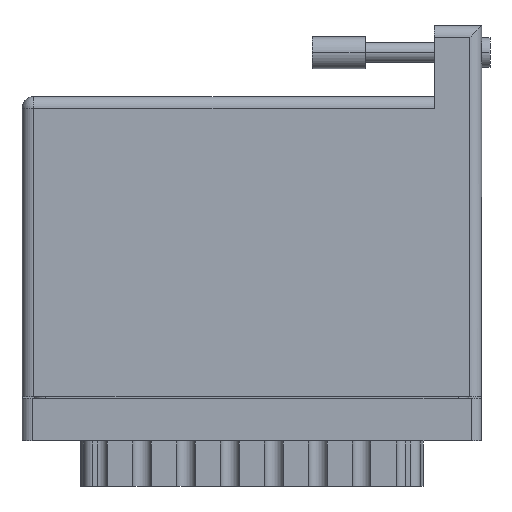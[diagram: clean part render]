
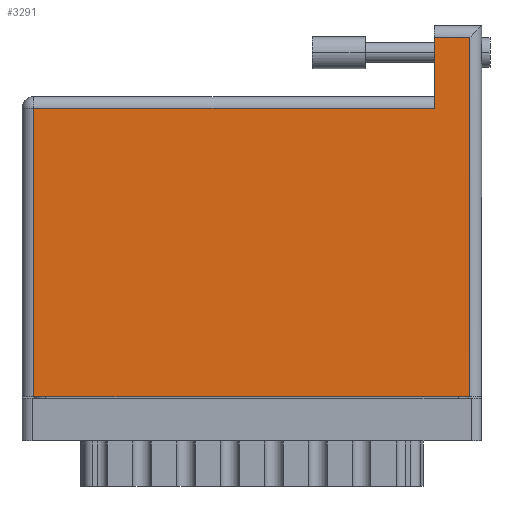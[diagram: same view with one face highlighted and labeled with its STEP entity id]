
A CAD part, front view. The second image highlights one B-rep face of the part: STEP entity #3291.
In plain terms, the highlighted face is planar.
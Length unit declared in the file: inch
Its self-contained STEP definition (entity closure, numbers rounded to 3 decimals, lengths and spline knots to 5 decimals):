
#130 = DIRECTION ( 'NONE',  ( -1., 0., 0. ) ) ;
#2239 = ORIENTED_EDGE ( 'NONE', *, *, #59741, .T. ) ;
#3291 = ADVANCED_FACE ( 'NONE', ( #67220 ), #52485, .F. ) ;
#6476 = CARTESIAN_POINT ( 'NONE',  ( 2.648, 0., 0. ) ) ;
#7361 = DIRECTION ( 'NONE',  ( 0., 0., -1. ) ) ;
#7433 = EDGE_LOOP ( 'NONE', ( #57592, #58185, #2239, #50515, #8734, #17443 ) ) ;
#8734 = ORIENTED_EDGE ( 'NONE', *, *, #58323, .T. ) ;
#8827 = EDGE_CURVE ( 'NONE', #49490, #54449, #51540, .T. ) ;
#10073 = CARTESIAN_POINT ( 'NONE',  ( 0., 1.705, 0. ) ) ;
#11583 = VERTEX_POINT ( 'NONE', #41017 ) ;
#15685 = DIRECTION ( 'NONE',  ( 0., -1., 0. ) ) ;
#17443 = ORIENTED_EDGE ( 'NONE', *, *, #55694, .T. ) ;
#17462 = EDGE_CURVE ( 'NONE', #61643, #49490, #47415, .T. ) ;
#17784 = DIRECTION ( 'NONE',  ( -1., 0., 0. ) ) ;
#19497 = EDGE_CURVE ( 'NONE', #45584, #11583, #55218, .T. ) ;
#20700 = VERTEX_POINT ( 'NONE', #58677 ) ;
#23329 = CARTESIAN_POINT ( 'NONE',  ( 0., 0., 0. ) ) ;
#23702 = LINE ( 'NONE', #65901, #54488 ) ;
#24988 = CARTESIAN_POINT ( 'NONE',  ( 0.07, 0., 0. ) ) ;
#28035 = VECTOR ( 'NONE', #15685, 39.37008 ) ;
#28466 = VECTOR ( 'NONE', #66991, 39.37008 ) ;
#31326 = CARTESIAN_POINT ( 'NONE',  ( 0.07, 0., 0. ) ) ;
#39415 = VECTOR ( 'NONE', #63774, 39.37008 ) ;
#41017 = CARTESIAN_POINT ( 'NONE',  ( 2.648, 2.125, 0. ) ) ;
#41182 = CARTESIAN_POINT ( 'NONE',  ( 2.438, 1.705, 0. ) ) ;
#42719 = CARTESIAN_POINT ( 'NONE',  ( 2.438, 2.195, 0. ) ) ;
#43372 = CARTESIAN_POINT ( 'NONE',  ( 0., 1.775, 0. ) ) ;
#44126 = DIRECTION ( 'NONE',  ( 1., 0., 0. ) ) ;
#45584 = VERTEX_POINT ( 'NONE', #6476 ) ;
#47415 = LINE ( 'NONE', #10073, #65191 ) ;
#48320 = LINE ( 'NONE', #42719, #39415 ) ;
#49490 = VERTEX_POINT ( 'NONE', #54366 ) ;
#50515 = ORIENTED_EDGE ( 'NONE', *, *, #19497, .T. ) ;
#51127 = LINE ( 'NONE', #23329, #64134 ) ;
#51540 = LINE ( 'NONE', #31326, #28035 ) ;
#52485 = PLANE ( 'NONE',  #66980 ) ;
#54366 = CARTESIAN_POINT ( 'NONE',  ( 0.07, 1.705, 0. ) ) ;
#54449 = VERTEX_POINT ( 'NONE', #24988 ) ;
#54488 = VECTOR ( 'NONE', #60951, 39.37008 ) ;
#55218 = LINE ( 'NONE', #61777, #28466 ) ;
#55694 = EDGE_CURVE ( 'NONE', #20700, #61643, #48320, .T. ) ;
#57592 = ORIENTED_EDGE ( 'NONE', *, *, #17462, .T. ) ;
#58185 = ORIENTED_EDGE ( 'NONE', *, *, #8827, .T. ) ;
#58323 = EDGE_CURVE ( 'NONE', #11583, #20700, #23702, .T. ) ;
#58677 = CARTESIAN_POINT ( 'NONE',  ( 2.438, 2.125, 0. ) ) ;
#59741 = EDGE_CURVE ( 'NONE', #54449, #45584, #51127, .T. ) ;
#60951 = DIRECTION ( 'NONE',  ( -1., 0., 0. ) ) ;
#61643 = VERTEX_POINT ( 'NONE', #41182 ) ;
#61777 = CARTESIAN_POINT ( 'NONE',  ( 2.648, 2.195, 0. ) ) ;
#63774 = DIRECTION ( 'NONE',  ( 0., -1., 0. ) ) ;
#64134 = VECTOR ( 'NONE', #44126, 39.37008 ) ;
#65191 = VECTOR ( 'NONE', #130, 39.37008 ) ;
#65901 = CARTESIAN_POINT ( 'NONE',  ( 0., 2.125, 0. ) ) ;
#66980 = AXIS2_PLACEMENT_3D ( 'NONE', #43372, #7361, #17784 ) ;
#66991 = DIRECTION ( 'NONE',  ( 0., 1., 0. ) ) ;
#67220 = FACE_OUTER_BOUND ( 'NONE', #7433, .T. ) ;
